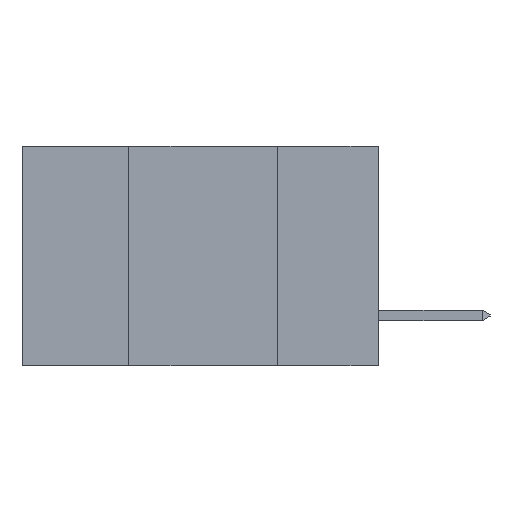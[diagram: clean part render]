
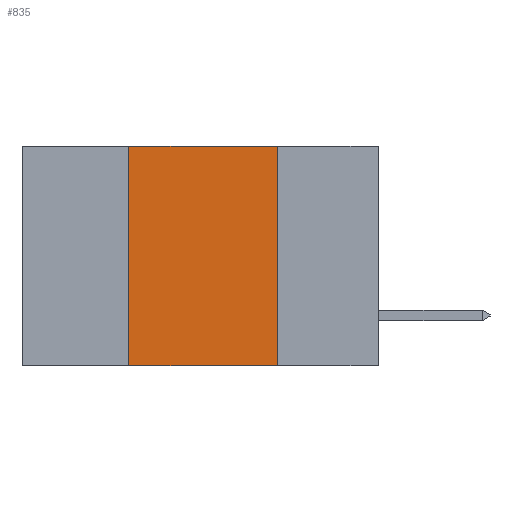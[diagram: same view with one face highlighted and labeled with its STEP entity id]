
A CAD part, left-side view. The second image highlights one B-rep face of the part: STEP entity #835.
In plain terms, the highlighted planar face has unit normal (-1, 0, 0).
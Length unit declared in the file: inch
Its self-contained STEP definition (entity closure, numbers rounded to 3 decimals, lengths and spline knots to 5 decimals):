
#835 = ADVANCED_FACE ( 'NONE', ( #5796 ), #6720, .F. ) ;
#1120 = EDGE_LOOP ( 'NONE', ( #2877, #3343, #1842, #1773 ) ) ;
#1211 = CARTESIAN_POINT ( 'NONE',  ( 0., 0.17, 0. ) ) ;
#1492 = VERTEX_POINT ( 'NONE', #4265 ) ;
#1773 = ORIENTED_EDGE ( 'NONE', *, *, #2938, .T. ) ;
#1842 = ORIENTED_EDGE ( 'NONE', *, *, #4362, .F. ) ;
#2058 = LINE ( 'NONE', #8948, #2726 ) ;
#2329 = VECTOR ( 'NONE', #7734, 39.37008 ) ;
#2340 = AXIS2_PLACEMENT_3D ( 'NONE', #6835, #7023, #7012 ) ;
#2716 = CARTESIAN_POINT ( 'NONE',  ( 0., 0.6, -0.37 ) ) ;
#2726 = VECTOR ( 'NONE', #3288, 39.37008 ) ;
#2877 = ORIENTED_EDGE ( 'NONE', *, *, #9915, .F. ) ;
#2938 = EDGE_CURVE ( 'NONE', #7149, #10709, #5369, .T. ) ;
#2979 = VERTEX_POINT ( 'NONE', #1211 ) ;
#3288 = DIRECTION ( 'NONE',  ( 0., 0., -1. ) ) ;
#3343 = ORIENTED_EDGE ( 'NONE', *, *, #9383, .F. ) ;
#4265 = CARTESIAN_POINT ( 'NONE',  ( 0., 0.42, 0. ) ) ;
#4362 = EDGE_CURVE ( 'NONE', #7149, #1492, #5324, .T. ) ;
#4610 = CARTESIAN_POINT ( 'NONE',  ( 0., 0.6, 0. ) ) ;
#4821 = LINE ( 'NONE', #4610, #11192 ) ;
#5324 = LINE ( 'NONE', #7571, #9765 ) ;
#5369 = LINE ( 'NONE', #2716, #2329 ) ;
#5796 = FACE_OUTER_BOUND ( 'NONE', #1120, .T. ) ;
#6720 = PLANE ( 'NONE',  #2340 ) ;
#6835 = CARTESIAN_POINT ( 'NONE',  ( 0., 0.6, 0. ) ) ;
#7012 = DIRECTION ( 'NONE',  ( 0., 0., -1. ) ) ;
#7023 = DIRECTION ( 'NONE',  ( 1., 0., 0. ) ) ;
#7149 = VERTEX_POINT ( 'NONE', #10770 ) ;
#7571 = CARTESIAN_POINT ( 'NONE',  ( 0., 0.42, -0.37 ) ) ;
#7586 = DIRECTION ( 'NONE',  ( 0., 0., 1. ) ) ;
#7734 = DIRECTION ( 'NONE',  ( 0., -1., 0. ) ) ;
#8948 = CARTESIAN_POINT ( 'NONE',  ( 0., 0.17, -0.37 ) ) ;
#9383 = EDGE_CURVE ( 'NONE', #1492, #2979, #4821, .T. ) ;
#9761 = CARTESIAN_POINT ( 'NONE',  ( 0., 0.17, -0.37 ) ) ;
#9765 = VECTOR ( 'NONE', #7586, 39.37008 ) ;
#9915 = EDGE_CURVE ( 'NONE', #2979, #10709, #2058, .T. ) ;
#10709 = VERTEX_POINT ( 'NONE', #9761 ) ;
#10770 = CARTESIAN_POINT ( 'NONE',  ( 0., 0.42, -0.37 ) ) ;
#11192 = VECTOR ( 'NONE', #11516, 39.37008 ) ;
#11516 = DIRECTION ( 'NONE',  ( 0., -1., 0. ) ) ;
